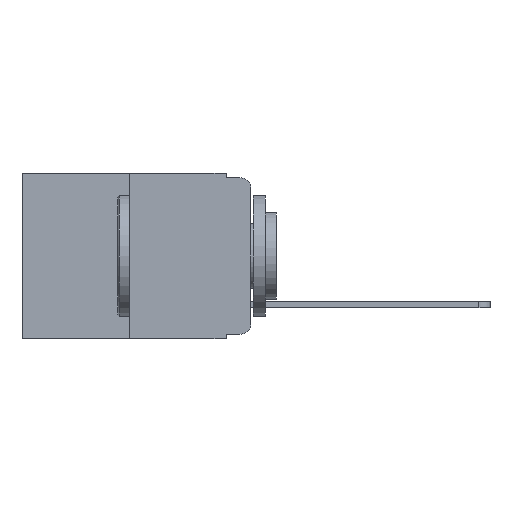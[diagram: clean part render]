
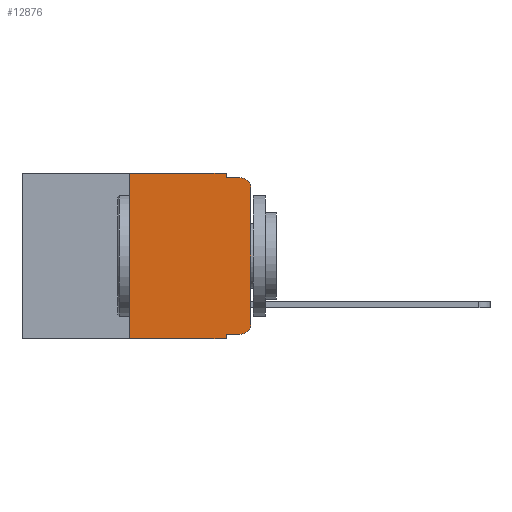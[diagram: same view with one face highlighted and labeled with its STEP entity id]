
A CAD part, left-side view. The second image highlights one B-rep face of the part: STEP entity #12876.
In plain terms, the highlighted planar face has unit normal (-1, 0, 0).
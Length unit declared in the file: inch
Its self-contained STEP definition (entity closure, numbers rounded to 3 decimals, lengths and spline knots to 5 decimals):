
#111 = VERTEX_POINT ( 'NONE', #7657 ) ;
#170 = DIRECTION ( 'NONE',  ( 0., -1., 0. ) ) ;
#389 = DIRECTION ( 'NONE',  ( 0., 0., -1. ) ) ;
#509 = VERTEX_POINT ( 'NONE', #944 ) ;
#588 = VECTOR ( 'NONE', #4116, 39.37008 ) ;
#944 = CARTESIAN_POINT ( 'NONE',  ( 0., 0., -0.313 ) ) ;
#1069 = EDGE_CURVE ( 'NONE', #4469, #509, #6896, .T. ) ;
#1511 = EDGE_CURVE ( 'NONE', #12858, #2339, #12933, .T. ) ;
#1518 = ORIENTED_EDGE ( 'NONE', *, *, #2760, .F. ) ;
#1526 = CARTESIAN_POINT ( 'NONE',  ( 0., 0.051, -0.01 ) ) ;
#1623 = EDGE_CURVE ( 'NONE', #2605, #2339, #11884, .T. ) ;
#1651 = ORIENTED_EDGE ( 'NONE', *, *, #2802, .T. ) ;
#2118 = ORIENTED_EDGE ( 'NONE', *, *, #5275, .T. ) ;
#2130 = DIRECTION ( 'NONE',  ( 0., -1., 0. ) ) ;
#2339 = VERTEX_POINT ( 'NONE', #11535 ) ;
#2384 = ORIENTED_EDGE ( 'NONE', *, *, #8016, .F. ) ;
#2388 = DIRECTION ( 'NONE',  ( 0., 0., 1. ) ) ;
#2476 = CARTESIAN_POINT ( 'NONE',  ( 0., 0.25, 0. ) ) ;
#2605 = VERTEX_POINT ( 'NONE', #8982 ) ;
#2760 = EDGE_CURVE ( 'NONE', #7268, #8475, #13268, .T. ) ;
#2790 = ORIENTED_EDGE ( 'NONE', *, *, #1511, .T. ) ;
#2802 = EDGE_CURVE ( 'NONE', #3551, #4469, #11041, .T. ) ;
#3551 = VERTEX_POINT ( 'NONE', #12660 ) ;
#3633 = VECTOR ( 'NONE', #9442, 39.37008 ) ;
#3869 = ORIENTED_EDGE ( 'NONE', *, *, #1623, .F. ) ;
#3916 = ORIENTED_EDGE ( 'NONE', *, *, #10057, .T. ) ;
#3968 = CARTESIAN_POINT ( 'NONE',  ( 0., 0.473, 0. ) ) ;
#4067 = VECTOR ( 'NONE', #2130, 39.37008 ) ;
#4116 = DIRECTION ( 'NONE',  ( 0., 0., 1. ) ) ;
#4147 = CARTESIAN_POINT ( 'NONE',  ( 0., 0., 0. ) ) ;
#4212 = EDGE_LOOP ( 'NONE', ( #2118, #2790, #3869, #11751, #1518, #2384, #3916, #11694, #1651, #12930 ) ) ;
#4306 = VERTEX_POINT ( 'NONE', #7199 ) ;
#4439 = AXIS2_PLACEMENT_3D ( 'NONE', #5440, #5057, #4605 ) ;
#4469 = VERTEX_POINT ( 'NONE', #9874 ) ;
#4605 = DIRECTION ( 'NONE',  ( 0., 0., -1. ) ) ;
#5057 = DIRECTION ( 'NONE',  ( -1., 0., 0. ) ) ;
#5254 = VECTOR ( 'NONE', #12117, 39.37008 ) ;
#5275 = EDGE_CURVE ( 'NONE', #509, #12858, #6792, .T. ) ;
#5440 = CARTESIAN_POINT ( 'NONE',  ( 0., 0.02, -0.03 ) ) ;
#5767 = FACE_OUTER_BOUND ( 'NONE', #4212, .T. ) ;
#5871 = VECTOR ( 'NONE', #2388, 39.37008 ) ;
#6157 = DIRECTION ( 'NONE',  ( 0., 0., -1. ) ) ;
#6325 = DIRECTION ( 'NONE',  ( -1., 0., 0. ) ) ;
#6331 = VECTOR ( 'NONE', #170, 39.37008 ) ;
#6792 = LINE ( 'NONE', #4147, #588 ) ;
#6896 = CIRCLE ( 'NONE', #7866, 0.02 ) ;
#7132 = CARTESIAN_POINT ( 'NONE',  ( 0., 0.473, -0.343 ) ) ;
#7160 = PLANE ( 'NONE',  #8592 ) ;
#7199 = CARTESIAN_POINT ( 'NONE',  ( 0., 0.25, -0.343 ) ) ;
#7268 = VERTEX_POINT ( 'NONE', #8073 ) ;
#7442 = LINE ( 'NONE', #9298, #9739 ) ;
#7657 = CARTESIAN_POINT ( 'NONE',  ( 0., 0.051, -0.343 ) ) ;
#7665 = EDGE_CURVE ( 'NONE', #3551, #111, #7996, .T. ) ;
#7866 = AXIS2_PLACEMENT_3D ( 'NONE', #13114, #6325, #9351 ) ;
#7996 = LINE ( 'NONE', #12439, #5254 ) ;
#8016 = EDGE_CURVE ( 'NONE', #4306, #7268, #11073, .T. ) ;
#8073 = CARTESIAN_POINT ( 'NONE',  ( 0., 0.25, 0. ) ) ;
#8101 = CARTESIAN_POINT ( 'NONE',  ( 0., 0., -0.03 ) ) ;
#8475 = VERTEX_POINT ( 'NONE', #9113 ) ;
#8592 = AXIS2_PLACEMENT_3D ( 'NONE', #3968, #11871, #6157 ) ;
#8982 = CARTESIAN_POINT ( 'NONE',  ( 0., 0.051, -0.01 ) ) ;
#9008 = LINE ( 'NONE', #7132, #6331 ) ;
#9113 = CARTESIAN_POINT ( 'NONE',  ( 0., 0.051, 0. ) ) ;
#9298 = CARTESIAN_POINT ( 'NONE',  ( 0., 0.051, 0. ) ) ;
#9351 = DIRECTION ( 'NONE',  ( 0., 0., -1. ) ) ;
#9396 = CARTESIAN_POINT ( 'NONE',  ( 0., 0.473, 0. ) ) ;
#9442 = DIRECTION ( 'NONE',  ( 0., -1., 0. ) ) ;
#9739 = VECTOR ( 'NONE', #389, 39.37008 ) ;
#9874 = CARTESIAN_POINT ( 'NONE',  ( 0., 0.02, -0.333 ) ) ;
#10057 = EDGE_CURVE ( 'NONE', #4306, #111, #9008, .T. ) ;
#10315 = EDGE_CURVE ( 'NONE', #8475, #2605, #7442, .T. ) ;
#10769 = VECTOR ( 'NONE', #12344, 39.37008 ) ;
#11041 = LINE ( 'NONE', #12406, #10769 ) ;
#11073 = LINE ( 'NONE', #2476, #5871 ) ;
#11535 = CARTESIAN_POINT ( 'NONE',  ( 0., 0.02, -0.01 ) ) ;
#11694 = ORIENTED_EDGE ( 'NONE', *, *, #7665, .F. ) ;
#11751 = ORIENTED_EDGE ( 'NONE', *, *, #10315, .F. ) ;
#11871 = DIRECTION ( 'NONE',  ( 1., 0., 0. ) ) ;
#11884 = LINE ( 'NONE', #1526, #4067 ) ;
#12117 = DIRECTION ( 'NONE',  ( 0., 0., -1. ) ) ;
#12344 = DIRECTION ( 'NONE',  ( 0., -1., 0. ) ) ;
#12406 = CARTESIAN_POINT ( 'NONE',  ( 0., 0.051, -0.333 ) ) ;
#12439 = CARTESIAN_POINT ( 'NONE',  ( 0., 0.051, 0. ) ) ;
#12660 = CARTESIAN_POINT ( 'NONE',  ( 0., 0.051, -0.333 ) ) ;
#12858 = VERTEX_POINT ( 'NONE', #8101 ) ;
#12876 = ADVANCED_FACE ( 'NONE', ( #5767 ), #7160, .F. ) ;
#12930 = ORIENTED_EDGE ( 'NONE', *, *, #1069, .T. ) ;
#12933 = CIRCLE ( 'NONE', #4439, 0.02 ) ;
#13114 = CARTESIAN_POINT ( 'NONE',  ( 0., 0.02, -0.313 ) ) ;
#13268 = LINE ( 'NONE', #9396, #3633 ) ;
